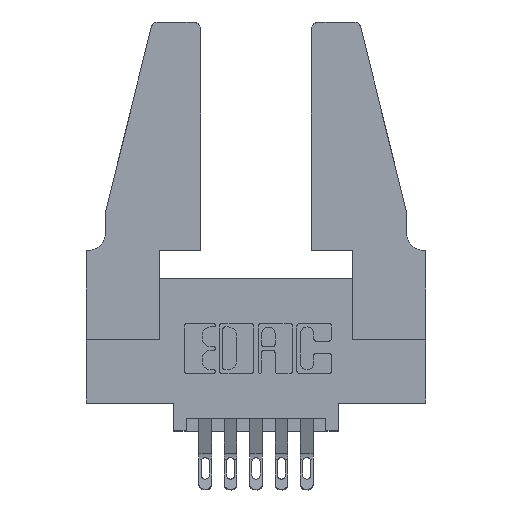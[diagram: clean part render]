
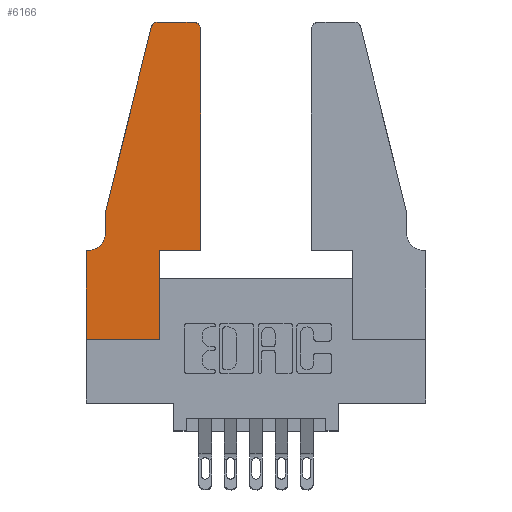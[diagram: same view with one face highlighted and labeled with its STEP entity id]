
A CAD part, top view. The second image highlights one B-rep face of the part: STEP entity #6166.
In plain terms, the highlighted planar face has unit normal (0, 0, 1).
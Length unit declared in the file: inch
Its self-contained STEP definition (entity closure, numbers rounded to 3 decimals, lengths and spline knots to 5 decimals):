
#48 = AXIS2_PLACEMENT_3D ( 'NONE', #1727, #751, #7133 ) ;
#230 = CARTESIAN_POINT ( 'NONE',  ( 0.2605, 1.25, 0.37 ) ) ;
#270 = ORIENTED_EDGE ( 'NONE', *, *, #10085, .T. ) ;
#295 = DIRECTION ( 'NONE',  ( -1., 0., 0. ) ) ;
#456 = CARTESIAN_POINT ( 'NONE',  ( 0.2865, 0., 0.37 ) ) ;
#499 = FACE_OUTER_BOUND ( 'NONE', #8967, .T. ) ;
#612 = EDGE_CURVE ( 'NONE', #7658, #10327, #2987, .T. ) ;
#676 = AXIS2_PLACEMENT_3D ( 'NONE', #1269, #6859, #8394 ) ;
#751 = DIRECTION ( 'NONE',  ( 0., 0., 1. ) ) ;
#815 = ORIENTED_EDGE ( 'NONE', *, *, #8049, .T. ) ;
#1114 = CARTESIAN_POINT ( 'NONE',  ( 0., 0., 0.37 ) ) ;
#1269 = CARTESIAN_POINT ( 'NONE',  ( 0.284, 1.22, 0.37 ) ) ;
#1284 = CARTESIAN_POINT ( 'NONE',  ( 0.4205, 1.25, 0.37 ) ) ;
#1317 = DIRECTION ( 'NONE',  ( 1., 0., 0. ) ) ;
#1665 = ORIENTED_EDGE ( 'NONE', *, *, #612, .T. ) ;
#1716 = DIRECTION ( 'NONE',  ( -0.239, -0.971, 0. ) ) ;
#1727 = CARTESIAN_POINT ( 'NONE',  ( 0.4205, 1.22, 0.37 ) ) ;
#1738 = EDGE_CURVE ( 'NONE', #2658, #7658, #2109, .T. ) ;
#1797 = ORIENTED_EDGE ( 'NONE', *, *, #9696, .T. ) ;
#1841 = CARTESIAN_POINT ( 'NONE',  ( 0.284, 1.25, 0.37 ) ) ;
#1874 = EDGE_CURVE ( 'NONE', #2329, #4204, #3907, .T. ) ;
#2009 = EDGE_CURVE ( 'NONE', #4204, #2658, #6585, .T. ) ;
#2055 = LINE ( 'NONE', #8250, #3463 ) ;
#2060 = DIRECTION ( 'NONE',  ( 0., 0., -1. ) ) ;
#2109 = LINE ( 'NONE', #5477, #7805 ) ;
#2236 = CARTESIAN_POINT ( 'NONE',  ( 0.0755, 0.5, 0.37 ) ) ;
#2329 = VERTEX_POINT ( 'NONE', #456 ) ;
#2427 = CIRCLE ( 'NONE', #8477, 0.07 ) ;
#2566 = CARTESIAN_POINT ( 'NONE',  ( 0.2865, 0.35, 0.37 ) ) ;
#2658 = VERTEX_POINT ( 'NONE', #2786 ) ;
#2786 = CARTESIAN_POINT ( 'NONE',  ( 0.4505, 0.35, 0.37 ) ) ;
#2788 = ORIENTED_EDGE ( 'NONE', *, *, #6113, .T. ) ;
#2946 = DIRECTION ( 'NONE',  ( 1., 0., 0. ) ) ;
#2987 = CIRCLE ( 'NONE', #48, 0.03 ) ;
#3133 = DIRECTION ( 'NONE',  ( 0., 0., 1. ) ) ;
#3397 = EDGE_CURVE ( 'NONE', #10248, #3982, #11449, .T. ) ;
#3435 = CARTESIAN_POINT ( 'NONE',  ( 0.0755, 0.5, 0.37 ) ) ;
#3463 = VECTOR ( 'NONE', #10033, 39.37008 ) ;
#3882 = LINE ( 'NONE', #230, #6540 ) ;
#3907 = LINE ( 'NONE', #2566, #5995 ) ;
#3982 = VERTEX_POINT ( 'NONE', #5994 ) ;
#4034 = VECTOR ( 'NONE', #4797, 39.37008 ) ;
#4086 = EDGE_CURVE ( 'NONE', #5008, #7178, #5456, .T. ) ;
#4204 = VERTEX_POINT ( 'NONE', #8183 ) ;
#4797 = DIRECTION ( 'NONE',  ( 0., -1., 0. ) ) ;
#4914 = EDGE_CURVE ( 'NONE', #7074, #8702, #6682, .T. ) ;
#5008 = VERTEX_POINT ( 'NONE', #10270 ) ;
#5080 = ORIENTED_EDGE ( 'NONE', *, *, #1738, .T. ) ;
#5148 = VERTEX_POINT ( 'NONE', #1114 ) ;
#5456 = LINE ( 'NONE', #10970, #9897 ) ;
#5477 = CARTESIAN_POINT ( 'NONE',  ( 0.4505, 0.35, 0.37 ) ) ;
#5574 = ORIENTED_EDGE ( 'NONE', *, *, #8144, .T. ) ;
#5600 = CARTESIAN_POINT ( 'NONE',  ( 0.0055, 0.42, 0.37 ) ) ;
#5994 = CARTESIAN_POINT ( 'NONE',  ( 0.25487, 1.22718, 0.37 ) ) ;
#5995 = VECTOR ( 'NONE', #7106, 39.37008 ) ;
#6113 = EDGE_CURVE ( 'NONE', #7178, #5148, #2055, .T. ) ;
#6128 = CARTESIAN_POINT ( 'NONE',  ( 0.0755, 0.5, 0.37 ) ) ;
#6166 = ADVANCED_FACE ( 'NONE', ( #499 ), #8530, .T. ) ;
#6246 = CARTESIAN_POINT ( 'NONE',  ( 0., 0.35, 0.37 ) ) ;
#6456 = CARTESIAN_POINT ( 'NONE',  ( 0.4505, 0.35, 0.37 ) ) ;
#6540 = VECTOR ( 'NONE', #8220, 39.37008 ) ;
#6585 = LINE ( 'NONE', #6456, #7267 ) ;
#6667 = DIRECTION ( 'NONE',  ( -1., 0., 0. ) ) ;
#6682 = LINE ( 'NONE', #2236, #4034 ) ;
#6725 = DIRECTION ( 'NONE',  ( 1., 0., 0. ) ) ;
#6836 = ORIENTED_EDGE ( 'NONE', *, *, #1874, .T. ) ;
#6859 = DIRECTION ( 'NONE',  ( 0., 0., 1. ) ) ;
#7074 = VERTEX_POINT ( 'NONE', #6128 ) ;
#7106 = DIRECTION ( 'NONE',  ( 0., 1., 0. ) ) ;
#7133 = DIRECTION ( 'NONE',  ( 1., 0., 0. ) ) ;
#7178 = VERTEX_POINT ( 'NONE', #6246 ) ;
#7267 = VECTOR ( 'NONE', #2946, 39.37008 ) ;
#7437 = ORIENTED_EDGE ( 'NONE', *, *, #4086, .T. ) ;
#7658 = VERTEX_POINT ( 'NONE', #11394 ) ;
#7697 = VECTOR ( 'NONE', #1317, 39.37008 ) ;
#7805 = VECTOR ( 'NONE', #8160, 39.37008 ) ;
#7902 = ORIENTED_EDGE ( 'NONE', *, *, #4914, .T. ) ;
#8016 = AXIS2_PLACEMENT_3D ( 'NONE', #11116, #3133, #6725 ) ;
#8049 = EDGE_CURVE ( 'NONE', #8702, #5008, #2427, .T. ) ;
#8144 = EDGE_CURVE ( 'NONE', #5148, #2329, #8418, .T. ) ;
#8160 = DIRECTION ( 'NONE',  ( 0., 1., 0. ) ) ;
#8183 = CARTESIAN_POINT ( 'NONE',  ( 0.2865, 0.35, 0.37 ) ) ;
#8220 = DIRECTION ( 'NONE',  ( -1., 0., 0. ) ) ;
#8250 = CARTESIAN_POINT ( 'NONE',  ( 0., 0., 0.37 ) ) ;
#8370 = CARTESIAN_POINT ( 'NONE',  ( 0., 0., 0.37 ) ) ;
#8394 = DIRECTION ( 'NONE',  ( 1., 0., 0. ) ) ;
#8418 = LINE ( 'NONE', #8370, #7697 ) ;
#8477 = AXIS2_PLACEMENT_3D ( 'NONE', #5600, #2060, #295 ) ;
#8530 = PLANE ( 'NONE',  #8016 ) ;
#8702 = VERTEX_POINT ( 'NONE', #10075 ) ;
#8967 = EDGE_LOOP ( 'NONE', ( #1797, #11053, #270, #7902, #815, #7437, #2788, #5574, #6836, #10569, #5080, #1665 ) ) ;
#9440 = VECTOR ( 'NONE', #1716, 39.37008 ) ;
#9696 = EDGE_CURVE ( 'NONE', #10327, #10248, #3882, .T. ) ;
#9897 = VECTOR ( 'NONE', #6667, 39.37008 ) ;
#10033 = DIRECTION ( 'NONE',  ( 0., -1., 0. ) ) ;
#10075 = CARTESIAN_POINT ( 'NONE',  ( 0.0755, 0.42, 0.37 ) ) ;
#10085 = EDGE_CURVE ( 'NONE', #3982, #7074, #11537, .T. ) ;
#10248 = VERTEX_POINT ( 'NONE', #1841 ) ;
#10270 = CARTESIAN_POINT ( 'NONE',  ( 0.0055, 0.35, 0.37 ) ) ;
#10327 = VERTEX_POINT ( 'NONE', #1284 ) ;
#10569 = ORIENTED_EDGE ( 'NONE', *, *, #2009, .T. ) ;
#10970 = CARTESIAN_POINT ( 'NONE',  ( 0.0755, 0.35, 0.37 ) ) ;
#11053 = ORIENTED_EDGE ( 'NONE', *, *, #3397, .T. ) ;
#11116 = CARTESIAN_POINT ( 'NONE',  ( 0., 0.35, 0.37 ) ) ;
#11394 = CARTESIAN_POINT ( 'NONE',  ( 0.4505, 1.22, 0.37 ) ) ;
#11449 = CIRCLE ( 'NONE', #676, 0.03 ) ;
#11537 = LINE ( 'NONE', #3435, #9440 ) ;
